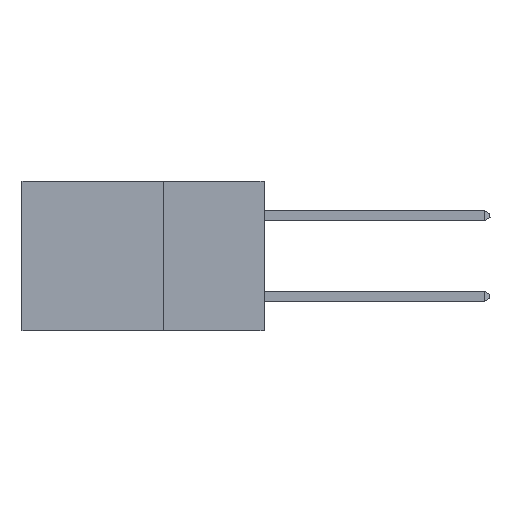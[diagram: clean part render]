
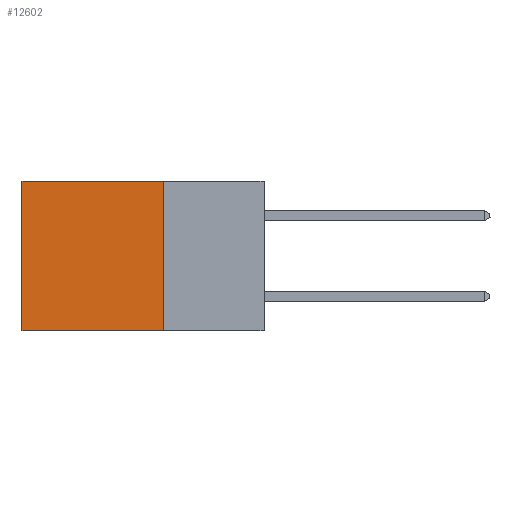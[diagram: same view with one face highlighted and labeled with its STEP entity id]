
A CAD part, left-side view. The second image highlights one B-rep face of the part: STEP entity #12602.
In plain terms, the highlighted planar face has unit normal (-1, 0, 0).
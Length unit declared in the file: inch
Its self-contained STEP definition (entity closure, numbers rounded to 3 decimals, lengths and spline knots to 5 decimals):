
#178 = CARTESIAN_POINT ( 'NONE',  ( 0.298, 0.25, 0. ) ) ;
#399 = CARTESIAN_POINT ( 'NONE',  ( 0.298, 0.25, 0. ) ) ;
#760 = VERTEX_POINT ( 'NONE', #3962 ) ;
#1129 = CARTESIAN_POINT ( 'NONE',  ( 0.298, 0.6, -0.37 ) ) ;
#1483 = VERTEX_POINT ( 'NONE', #178 ) ;
#1651 = DIRECTION ( 'NONE',  ( 0., 0., -1. ) ) ;
#2486 = VECTOR ( 'NONE', #1651, 39.37008 ) ;
#2624 = EDGE_CURVE ( 'NONE', #3702, #5698, #14151, .T. ) ;
#2704 = ORIENTED_EDGE ( 'NONE', *, *, #6402, .T. ) ;
#2747 = ORIENTED_EDGE ( 'NONE', *, *, #2624, .F. ) ;
#2935 = CARTESIAN_POINT ( 'NONE',  ( 0.298, 0.6, 0. ) ) ;
#3702 = VERTEX_POINT ( 'NONE', #14176 ) ;
#3962 = CARTESIAN_POINT ( 'NONE',  ( 0.298, 0.6, 0. ) ) ;
#4282 = CARTESIAN_POINT ( 'NONE',  ( 0.298, 0.25, 0. ) ) ;
#5575 = AXIS2_PLACEMENT_3D ( 'NONE', #6157, #12299, #9800 ) ;
#5698 = VERTEX_POINT ( 'NONE', #1129 ) ;
#5705 = LINE ( 'NONE', #4282, #2486 ) ;
#5944 = EDGE_CURVE ( 'NONE', #1483, #3702, #5705, .T. ) ;
#6157 = CARTESIAN_POINT ( 'NONE',  ( 0.298, 0.25, 0. ) ) ;
#6402 = EDGE_CURVE ( 'NONE', #1483, #760, #9901, .T. ) ;
#7301 = FACE_OUTER_BOUND ( 'NONE', #15131, .T. ) ;
#8014 = CARTESIAN_POINT ( 'NONE',  ( 0.298, 0.25, -0.37 ) ) ;
#8659 = ORIENTED_EDGE ( 'NONE', *, *, #5944, .F. ) ;
#9054 = DIRECTION ( 'NONE',  ( 0., 0., -1. ) ) ;
#9800 = DIRECTION ( 'NONE',  ( 0., 0., -1. ) ) ;
#9901 = LINE ( 'NONE', #399, #12357 ) ;
#9938 = ORIENTED_EDGE ( 'NONE', *, *, #14948, .T. ) ;
#10265 = VECTOR ( 'NONE', #9054, 39.37008 ) ;
#10895 = VECTOR ( 'NONE', #15240, 39.37008 ) ;
#11183 = PLANE ( 'NONE',  #5575 ) ;
#11386 = DIRECTION ( 'NONE',  ( 0., 1., 0. ) ) ;
#11808 = LINE ( 'NONE', #2935, #10265 ) ;
#12299 = DIRECTION ( 'NONE',  ( 1., 0., 0. ) ) ;
#12357 = VECTOR ( 'NONE', #11386, 39.37008 ) ;
#12602 = ADVANCED_FACE ( 'NONE', ( #7301 ), #11183, .F. ) ;
#14151 = LINE ( 'NONE', #8014, #10895 ) ;
#14176 = CARTESIAN_POINT ( 'NONE',  ( 0.298, 0.25, -0.37 ) ) ;
#14948 = EDGE_CURVE ( 'NONE', #760, #5698, #11808, .T. ) ;
#15131 = EDGE_LOOP ( 'NONE', ( #9938, #2747, #8659, #2704 ) ) ;
#15240 = DIRECTION ( 'NONE',  ( 0., 1., 0. ) ) ;
